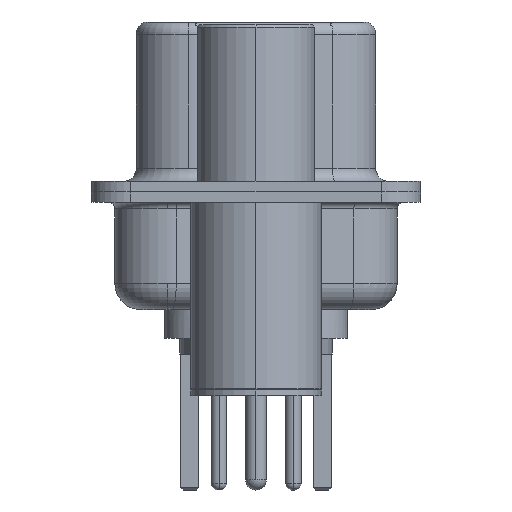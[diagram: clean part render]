
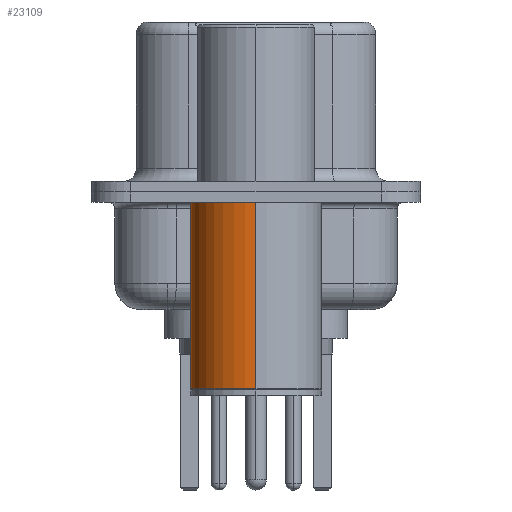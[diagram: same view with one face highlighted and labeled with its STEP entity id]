
A CAD part, left-side view. The second image highlights one B-rep face of the part: STEP entity #23109.
In plain terms, the highlighted cylindrical face has radius 2.5 mm (diameter 5 mm), a partial arc.
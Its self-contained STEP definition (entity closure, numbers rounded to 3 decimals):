
#13 = DIRECTION ( 'NONE',  ( 0., 0., 1. ) ) ;
#290 = DIRECTION ( 'NONE',  ( 0., 0., 1. ) ) ;
#578 = CYLINDRICAL_SURFACE ( 'NONE', #13681, 2.5 ) ;
#732 = ORIENTED_EDGE ( 'NONE', *, *, #22163, .F. ) ;
#1522 = DIRECTION ( 'NONE',  ( 1., 0., 0. ) ) ;
#2417 = ORIENTED_EDGE ( 'NONE', *, *, #5310, .T. ) ;
#4839 = CARTESIAN_POINT ( 'NONE',  ( -2.5, 0., -7.525 ) ) ;
#5310 = EDGE_CURVE ( 'NONE', #8031, #8462, #9132, .T. ) ;
#6284 = CARTESIAN_POINT ( 'NONE',  ( 2.5, 0., -7.525 ) ) ;
#8031 = VERTEX_POINT ( 'NONE', #4839 ) ;
#8462 = VERTEX_POINT ( 'NONE', #12069 ) ;
#9132 = LINE ( 'NONE', #11214, #14669 ) ;
#9858 = LINE ( 'NONE', #13150, #21647 ) ;
#9993 = DIRECTION ( 'NONE',  ( 0., 0., 1. ) ) ;
#10277 = ORIENTED_EDGE ( 'NONE', *, *, #17584, .T. ) ;
#10974 = CIRCLE ( 'NONE', #13909, 2.5 ) ;
#11002 = ORIENTED_EDGE ( 'NONE', *, *, #20152, .F. ) ;
#11214 = CARTESIAN_POINT ( 'NONE',  ( -2.5, 0., 0.581 ) ) ;
#11752 = FACE_OUTER_BOUND ( 'NONE', #20196, .T. ) ;
#12069 = CARTESIAN_POINT ( 'NONE',  ( -2.5, 0., -0.4 ) ) ;
#12868 = CARTESIAN_POINT ( 'NONE',  ( 0., 0., -0.4 ) ) ;
#13150 = CARTESIAN_POINT ( 'NONE',  ( 2.5, 0., 0.581 ) ) ;
#13681 = AXIS2_PLACEMENT_3D ( 'NONE', #14070, #18154, #1522 ) ;
#13909 = AXIS2_PLACEMENT_3D ( 'NONE', #22526, #9993, #24652 ) ;
#14070 = CARTESIAN_POINT ( 'NONE',  ( 0., 0., 0.581 ) ) ;
#14669 = VECTOR ( 'NONE', #13, 1000. ) ;
#14958 = DIRECTION ( 'NONE',  ( 1., 0., 0. ) ) ;
#17584 = EDGE_CURVE ( 'NONE', #23853, #8031, #10974, .T. ) ;
#18154 = DIRECTION ( 'NONE',  ( 0., 0., 1. ) ) ;
#19348 = DIRECTION ( 'NONE',  ( 0., 0., 1. ) ) ;
#20152 = EDGE_CURVE ( 'NONE', #23853, #20199, #9858, .T. ) ;
#20196 = EDGE_LOOP ( 'NONE', ( #10277, #2417, #732, #11002 ) ) ;
#20199 = VERTEX_POINT ( 'NONE', #23675 ) ;
#21647 = VECTOR ( 'NONE', #19348, 1000. ) ;
#22163 = EDGE_CURVE ( 'NONE', #20199, #8462, #23914, .T. ) ;
#22526 = CARTESIAN_POINT ( 'NONE',  ( 0., 0., -7.525 ) ) ;
#22768 = AXIS2_PLACEMENT_3D ( 'NONE', #12868, #290, #14958 ) ;
#23109 = ADVANCED_FACE ( 'NONE', ( #11752 ), #578, .T. ) ;
#23675 = CARTESIAN_POINT ( 'NONE',  ( 2.5, 0., -0.4 ) ) ;
#23853 = VERTEX_POINT ( 'NONE', #6284 ) ;
#23914 = CIRCLE ( 'NONE', #22768, 2.5 ) ;
#24652 = DIRECTION ( 'NONE',  ( 1., 0., 0. ) ) ;
